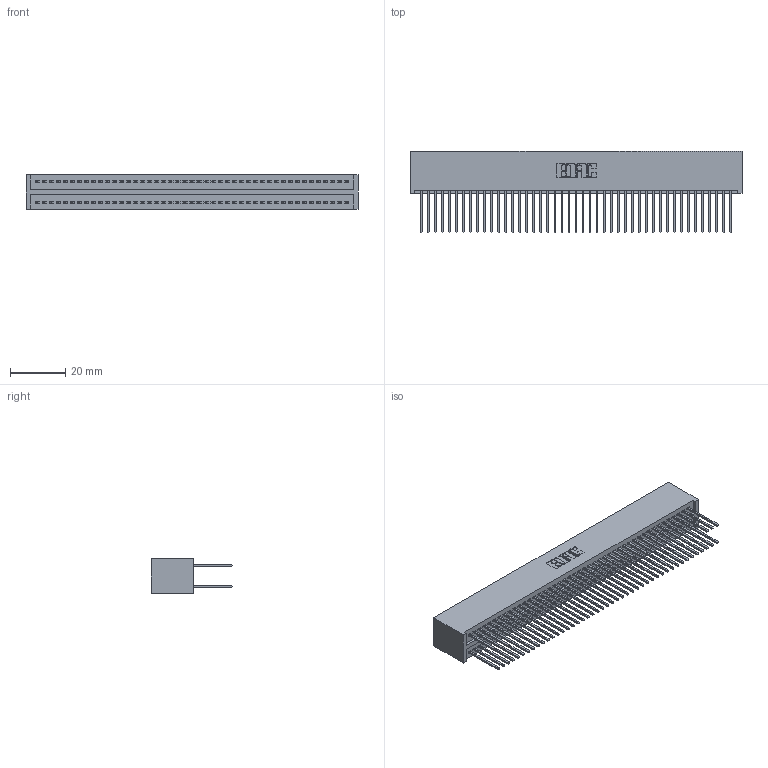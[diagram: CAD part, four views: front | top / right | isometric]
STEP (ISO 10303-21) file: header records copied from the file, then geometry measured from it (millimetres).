
FILE_DESCRIPTION (( 'STEP AP203' ), '1' );
FILE_NAME ('325-090-540-201.STEP', '2020-02-25T05:40:30', ( '' ), ( '' ), 'SwSTEP 2.0', 'SolidWorks 2016', '' );
FILE_SCHEMA (( 'CONFIG_CONTROL_DESIGN' ));
Length unit declared in the file: inch
Products named in the file (3): 325-090-540-201; 325 Part_Lugless; 325-292-001_325-293-140
Assembly tree (91 placements, depth 2):
  325-090-540-201
    325 Part_Lugless
    325-292-001_325-293-140  x90
Bounding box: 119.94 x 29.46 x 12.45 mm (x, y, z)
Volume: 16458.1 mm3; surface area: 22276.5 mm2
Topology: 91 solids, 91 shells, 4786 faces, 14237 edges, 9370 vertices
Faces by surface type: plane 3306, cylinder 1480
Entity records: 28303 total; most frequent: CARTESIAN_POINT 4686, ORIENTED_EDGE 4622, DIRECTION 3991, EDGE_CURVE 2311, LINE 2191, VECTOR 2191, VERTEX_POINT 1538, AXIS2_PLACEMENT_3D 900
